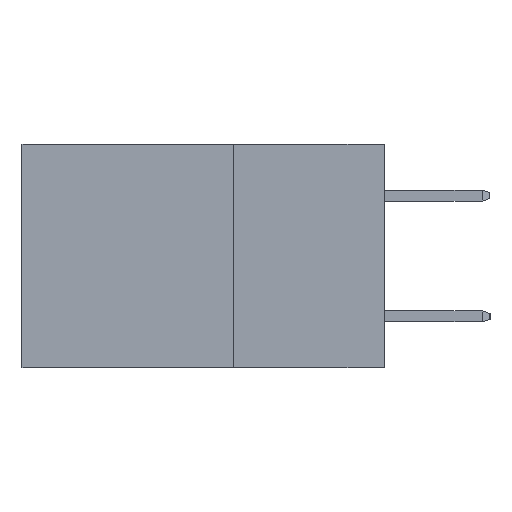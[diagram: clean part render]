
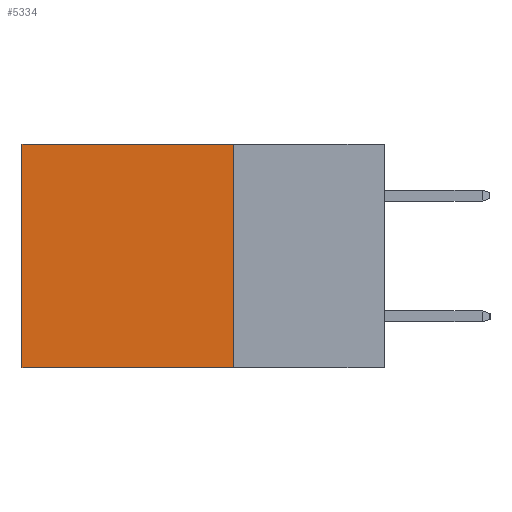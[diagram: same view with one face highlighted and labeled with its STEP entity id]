
A CAD part, left-side view. The second image highlights one B-rep face of the part: STEP entity #5334.
In plain terms, the highlighted planar face has unit normal (-1, 0, 0).
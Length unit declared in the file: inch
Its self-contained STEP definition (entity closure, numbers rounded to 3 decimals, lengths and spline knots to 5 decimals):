
#49 = EDGE_CURVE ( 'NONE', #1954, #9709, #9290, .T. ) ;
#99 = VECTOR ( 'NONE', #1927, 39.37008 ) ;
#839 = LINE ( 'NONE', #1333, #4827 ) ;
#1041 = EDGE_CURVE ( 'NONE', #9012, #1401, #4443, .T. ) ;
#1270 = DIRECTION ( 'NONE',  ( 0., 0., -1. ) ) ;
#1333 = CARTESIAN_POINT ( 'NONE',  ( 0.2615, 0.25, -0.37 ) ) ;
#1401 = VERTEX_POINT ( 'NONE', #1864 ) ;
#1762 = CARTESIAN_POINT ( 'NONE',  ( 0.2615, 0.25, 0. ) ) ;
#1864 = CARTESIAN_POINT ( 'NONE',  ( 0.2615, 0.6, -0.37 ) ) ;
#1927 = DIRECTION ( 'NONE',  ( 0., 1., 0. ) ) ;
#1954 = VERTEX_POINT ( 'NONE', #1762 ) ;
#2011 = CARTESIAN_POINT ( 'NONE',  ( 0.2615, 0.25, -0.37 ) ) ;
#3415 = ORIENTED_EDGE ( 'NONE', *, *, #5410, .T. ) ;
#3493 = CARTESIAN_POINT ( 'NONE',  ( 0.2615, 0.6, 0. ) ) ;
#3918 = EDGE_LOOP ( 'NONE', ( #3415, #4782, #7682, #8533 ) ) ;
#4383 = EDGE_CURVE ( 'NONE', #1954, #9012, #839, .T. ) ;
#4443 = LINE ( 'NONE', #2011, #99 ) ;
#4782 = ORIENTED_EDGE ( 'NONE', *, *, #1041, .F. ) ;
#4827 = VECTOR ( 'NONE', #1270, 39.37008 ) ;
#4897 = VECTOR ( 'NONE', #6881, 39.37008 ) ;
#5126 = LINE ( 'NONE', #6871, #4897 ) ;
#5218 = CARTESIAN_POINT ( 'NONE',  ( 0.2615, 0.25, -0.37 ) ) ;
#5233 = DIRECTION ( 'NONE',  ( 0., 1., 0. ) ) ;
#5334 = ADVANCED_FACE ( 'NONE', ( #9178 ), #7135, .F. ) ;
#5410 = EDGE_CURVE ( 'NONE', #9709, #1401, #5126, .T. ) ;
#6206 = DIRECTION ( 'NONE',  ( 1., 0., 0. ) ) ;
#6245 = DIRECTION ( 'NONE',  ( 0., 0., -1. ) ) ;
#6871 = CARTESIAN_POINT ( 'NONE',  ( 0.2615, 0.6, -0.37 ) ) ;
#6881 = DIRECTION ( 'NONE',  ( 0., 0., -1. ) ) ;
#7089 = CARTESIAN_POINT ( 'NONE',  ( 0.2615, 0.25, -0.37 ) ) ;
#7098 = CARTESIAN_POINT ( 'NONE',  ( 0.2615, 0.25, 0. ) ) ;
#7135 = PLANE ( 'NONE',  #8700 ) ;
#7682 = ORIENTED_EDGE ( 'NONE', *, *, #4383, .F. ) ;
#8533 = ORIENTED_EDGE ( 'NONE', *, *, #49, .T. ) ;
#8700 = AXIS2_PLACEMENT_3D ( 'NONE', #7089, #6206, #6245 ) ;
#9012 = VERTEX_POINT ( 'NONE', #5218 ) ;
#9079 = VECTOR ( 'NONE', #5233, 39.37008 ) ;
#9178 = FACE_OUTER_BOUND ( 'NONE', #3918, .T. ) ;
#9290 = LINE ( 'NONE', #7098, #9079 ) ;
#9709 = VERTEX_POINT ( 'NONE', #3493 ) ;
